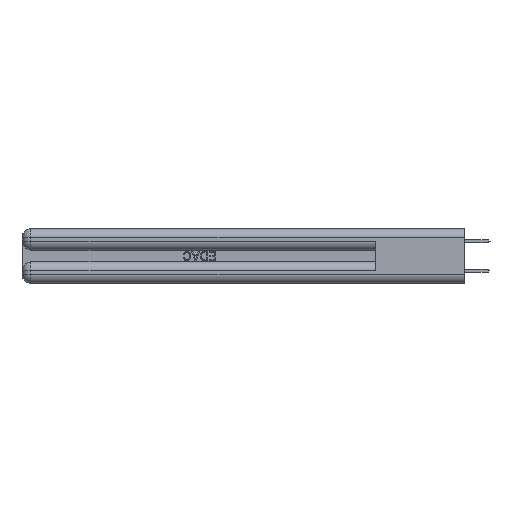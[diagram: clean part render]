
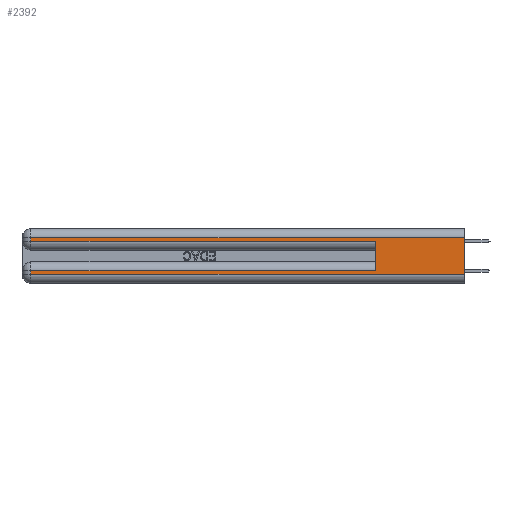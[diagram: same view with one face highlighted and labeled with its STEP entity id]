
A CAD part, left-side view. The second image highlights one B-rep face of the part: STEP entity #2392.
In plain terms, the highlighted planar face has unit normal (-1, 0, 0).
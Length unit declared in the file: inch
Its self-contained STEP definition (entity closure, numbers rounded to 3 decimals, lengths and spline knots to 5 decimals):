
#506 = VERTEX_POINT ( 'NONE', #18205 ) ;
#537 = CARTESIAN_POINT ( 'NONE',  ( 0., 0., 0.37 ) ) ;
#2392 = ADVANCED_FACE ( 'NONE', ( #25128 ), #23093, .F. ) ;
#3971 = EDGE_CURVE ( 'NONE', #37756, #506, #40176, .T. ) ;
#4204 = VECTOR ( 'NONE', #8602, 39.37008 ) ;
#5720 = DIRECTION ( 'NONE',  ( 0., 0., -1. ) ) ;
#6322 = VECTOR ( 'NONE', #26855, 39.37008 ) ;
#7062 = CARTESIAN_POINT ( 'NONE',  ( 0., 2.94, 0.285 ) ) ;
#7385 = CARTESIAN_POINT ( 'NONE',  ( 0., 0., 0.06 ) ) ;
#7494 = DIRECTION ( 'NONE',  ( 0., -1., 0. ) ) ;
#8540 = VERTEX_POINT ( 'NONE', #41228 ) ;
#8602 = DIRECTION ( 'NONE',  ( 0., 1., 0. ) ) ;
#8890 = DIRECTION ( 'NONE',  ( 0., 0., -1. ) ) ;
#9136 = EDGE_CURVE ( 'NONE', #37756, #37597, #15039, .T. ) ;
#9183 = DIRECTION ( 'NONE',  ( 1., 0., 0. ) ) ;
#9681 = ORIENTED_EDGE ( 'NONE', *, *, #3971, .F. ) ;
#12110 = LINE ( 'NONE', #16370, #22937 ) ;
#12642 = EDGE_CURVE ( 'NONE', #24432, #23322, #41209, .T. ) ;
#13547 = LINE ( 'NONE', #18863, #40100 ) ;
#13575 = VECTOR ( 'NONE', #28730, 39.37008 ) ;
#15039 = LINE ( 'NONE', #37316, #6322 ) ;
#16370 = CARTESIAN_POINT ( 'NONE',  ( 0., 0., 0.285 ) ) ;
#16616 = CARTESIAN_POINT ( 'NONE',  ( 0., 2.94, 0.085 ) ) ;
#17353 = CARTESIAN_POINT ( 'NONE',  ( 0., 0.6, 0.085 ) ) ;
#18205 = CARTESIAN_POINT ( 'NONE',  ( 0., 0.6, 0.285 ) ) ;
#18392 = EDGE_CURVE ( 'NONE', #26032, #23322, #21733, .T. ) ;
#18863 = CARTESIAN_POINT ( 'NONE',  ( 0., 2.94, 0.37 ) ) ;
#20858 = ORIENTED_EDGE ( 'NONE', *, *, #40325, .T. ) ;
#21077 = LINE ( 'NONE', #36719, #25462 ) ;
#21181 = VECTOR ( 'NONE', #7494, 39.37008 ) ;
#21733 = LINE ( 'NONE', #38379, #21181 ) ;
#22937 = VECTOR ( 'NONE', #40546, 39.37008 ) ;
#23093 = PLANE ( 'NONE',  #33171 ) ;
#23322 = VERTEX_POINT ( 'NONE', #7385 ) ;
#23482 = CARTESIAN_POINT ( 'NONE',  ( 0., 0., 0.31 ) ) ;
#23885 = ORIENTED_EDGE ( 'NONE', *, *, #27306, .T. ) ;
#24158 = LINE ( 'NONE', #29302, #4204 ) ;
#24432 = VERTEX_POINT ( 'NONE', #23482 ) ;
#25128 = FACE_OUTER_BOUND ( 'NONE', #38817, .T. ) ;
#25363 = EDGE_CURVE ( 'NONE', #37597, #26032, #13547, .T. ) ;
#25462 = VECTOR ( 'NONE', #8890, 39.37008 ) ;
#26032 = VERTEX_POINT ( 'NONE', #43075 ) ;
#26855 = DIRECTION ( 'NONE',  ( 0., 1., 0. ) ) ;
#27306 = EDGE_CURVE ( 'NONE', #8540, #43201, #21077, .T. ) ;
#28730 = DIRECTION ( 'NONE',  ( 0., 0., -1. ) ) ;
#29302 = CARTESIAN_POINT ( 'NONE',  ( 0., 0., 0.31 ) ) ;
#29850 = ORIENTED_EDGE ( 'NONE', *, *, #9136, .T. ) ;
#30439 = CARTESIAN_POINT ( 'NONE',  ( 0., 0., 0.37 ) ) ;
#31217 = CARTESIAN_POINT ( 'NONE',  ( 0., 0.6, 0.145 ) ) ;
#31831 = DIRECTION ( 'NONE',  ( 0., 0., 1. ) ) ;
#33171 = AXIS2_PLACEMENT_3D ( 'NONE', #30439, #9183, #5720 ) ;
#36427 = ORIENTED_EDGE ( 'NONE', *, *, #12642, .F. ) ;
#36719 = CARTESIAN_POINT ( 'NONE',  ( 0., 2.94, 0.37 ) ) ;
#37316 = CARTESIAN_POINT ( 'NONE',  ( 0., 0., 0.085 ) ) ;
#37597 = VERTEX_POINT ( 'NONE', #16616 ) ;
#37682 = ORIENTED_EDGE ( 'NONE', *, *, #18392, .T. ) ;
#37756 = VERTEX_POINT ( 'NONE', #17353 ) ;
#38286 = ORIENTED_EDGE ( 'NONE', *, *, #42132, .T. ) ;
#38379 = CARTESIAN_POINT ( 'NONE',  ( 0., 0., 0.06 ) ) ;
#38817 = EDGE_LOOP ( 'NONE', ( #36427, #20858, #23885, #38286, #9681, #29850, #39296, #37682 ) ) ;
#39296 = ORIENTED_EDGE ( 'NONE', *, *, #25363, .T. ) ;
#39745 = DIRECTION ( 'NONE',  ( 0., 0., -1. ) ) ;
#40100 = VECTOR ( 'NONE', #39745, 39.37008 ) ;
#40176 = LINE ( 'NONE', #31217, #40696 ) ;
#40325 = EDGE_CURVE ( 'NONE', #24432, #8540, #24158, .T. ) ;
#40546 = DIRECTION ( 'NONE',  ( 0., -1., 0. ) ) ;
#40696 = VECTOR ( 'NONE', #31831, 39.37008 ) ;
#41209 = LINE ( 'NONE', #537, #13575 ) ;
#41228 = CARTESIAN_POINT ( 'NONE',  ( 0., 2.94, 0.31 ) ) ;
#42132 = EDGE_CURVE ( 'NONE', #43201, #506, #12110, .T. ) ;
#43075 = CARTESIAN_POINT ( 'NONE',  ( 0., 2.94, 0.06 ) ) ;
#43201 = VERTEX_POINT ( 'NONE', #7062 ) ;
